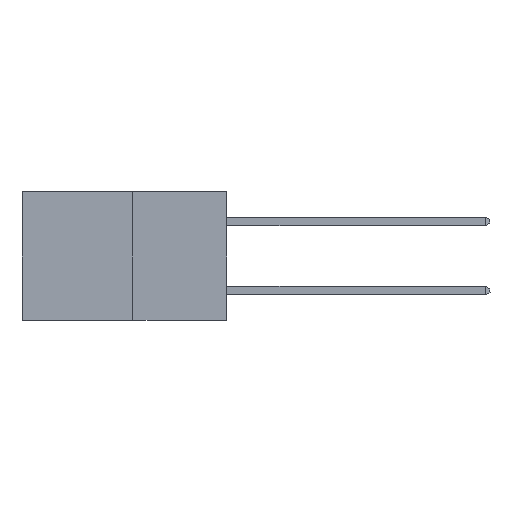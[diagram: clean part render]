
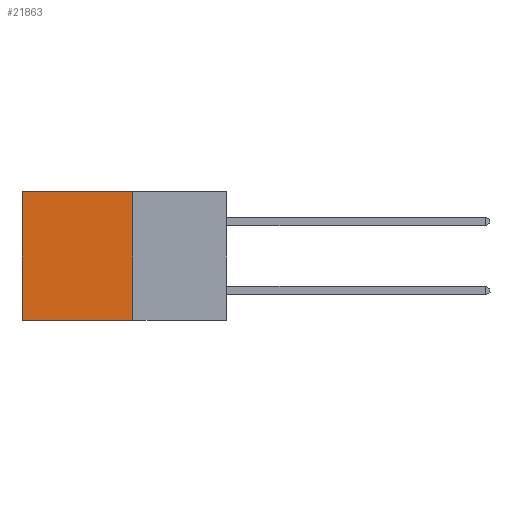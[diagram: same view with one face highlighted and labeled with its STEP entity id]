
A CAD part, left-side view. The second image highlights one B-rep face of the part: STEP entity #21863.
In plain terms, the highlighted planar face has unit normal (-1, 0, 0).
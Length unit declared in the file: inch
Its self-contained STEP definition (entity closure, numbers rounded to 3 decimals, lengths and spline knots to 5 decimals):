
#200 = VECTOR ( 'NONE', #3742, 39.37008 ) ;
#909 = VERTEX_POINT ( 'NONE', #14091 ) ;
#1476 = CARTESIAN_POINT ( 'NONE',  ( 0.277, 0.27, -0.37 ) ) ;
#2647 = CARTESIAN_POINT ( 'NONE',  ( 0.277, 0.27, -0.37 ) ) ;
#3033 = ORIENTED_EDGE ( 'NONE', *, *, #4238, .F. ) ;
#3332 = PLANE ( 'NONE',  #6399 ) ;
#3742 = DIRECTION ( 'NONE',  ( 0., 1., 0. ) ) ;
#4132 = CARTESIAN_POINT ( 'NONE',  ( 0.277, 0.27, 0. ) ) ;
#4159 = EDGE_LOOP ( 'NONE', ( #22235, #8689, #3033, #16652 ) ) ;
#4238 = EDGE_CURVE ( 'NONE', #10007, #12064, #20889, .T. ) ;
#4675 = CARTESIAN_POINT ( 'NONE',  ( 0.277, 0.59, -0.37 ) ) ;
#5528 = VECTOR ( 'NONE', #18012, 39.37008 ) ;
#5574 = EDGE_CURVE ( 'NONE', #909, #17747, #20071, .T. ) ;
#5719 = EDGE_CURVE ( 'NONE', #12064, #17747, #16689, .T. ) ;
#6399 = AXIS2_PLACEMENT_3D ( 'NONE', #1476, #19816, #8949 ) ;
#7013 = CARTESIAN_POINT ( 'NONE',  ( 0.277, 0.27, -0.37 ) ) ;
#7943 = EDGE_CURVE ( 'NONE', #10007, #909, #19696, .T. ) ;
#8689 = ORIENTED_EDGE ( 'NONE', *, *, #5719, .F. ) ;
#8823 = DIRECTION ( 'NONE',  ( 0., 1., 0. ) ) ;
#8949 = DIRECTION ( 'NONE',  ( 0., 0., -1. ) ) ;
#10007 = VERTEX_POINT ( 'NONE', #20856 ) ;
#11878 = VECTOR ( 'NONE', #8823, 39.37008 ) ;
#12064 = VERTEX_POINT ( 'NONE', #2647 ) ;
#14091 = CARTESIAN_POINT ( 'NONE',  ( 0.277, 0.59, 0. ) ) ;
#16118 = VECTOR ( 'NONE', #16870, 39.37008 ) ;
#16652 = ORIENTED_EDGE ( 'NONE', *, *, #7943, .T. ) ;
#16689 = LINE ( 'NONE', #7013, #11878 ) ;
#16870 = DIRECTION ( 'NONE',  ( 0., 0., -1. ) ) ;
#17747 = VERTEX_POINT ( 'NONE', #4675 ) ;
#18012 = DIRECTION ( 'NONE',  ( 0., 0., -1. ) ) ;
#18534 = CARTESIAN_POINT ( 'NONE',  ( 0.277, 0.59, -0.37 ) ) ;
#18894 = FACE_OUTER_BOUND ( 'NONE', #4159, .T. ) ;
#19068 = CARTESIAN_POINT ( 'NONE',  ( 0.277, 0.27, -0.37 ) ) ;
#19696 = LINE ( 'NONE', #4132, #200 ) ;
#19816 = DIRECTION ( 'NONE',  ( 1., 0., 0. ) ) ;
#20071 = LINE ( 'NONE', #18534, #5528 ) ;
#20856 = CARTESIAN_POINT ( 'NONE',  ( 0.277, 0.27, 0. ) ) ;
#20889 = LINE ( 'NONE', #19068, #16118 ) ;
#21863 = ADVANCED_FACE ( 'NONE', ( #18894 ), #3332, .F. ) ;
#22235 = ORIENTED_EDGE ( 'NONE', *, *, #5574, .T. ) ;
